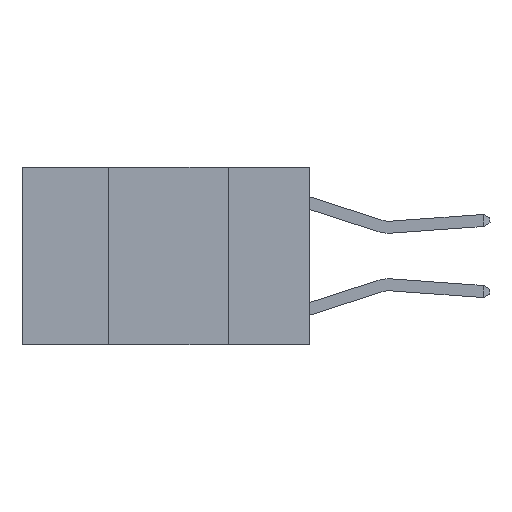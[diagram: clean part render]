
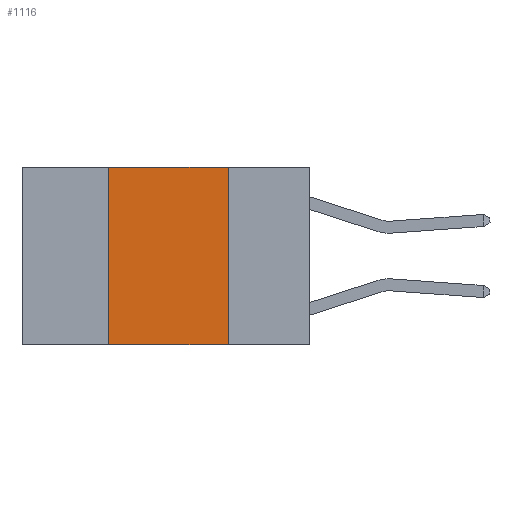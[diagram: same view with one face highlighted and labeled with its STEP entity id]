
A CAD part, left-side view. The second image highlights one B-rep face of the part: STEP entity #1116.
In plain terms, the highlighted planar face has unit normal (-1, 0, 0).
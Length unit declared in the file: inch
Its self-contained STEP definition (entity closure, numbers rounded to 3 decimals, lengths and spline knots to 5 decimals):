
#215 = CARTESIAN_POINT ( 'NONE',  ( 0., 0.6, 0. ) ) ;
#395 = FACE_OUTER_BOUND ( 'NONE', #25441, .T. ) ;
#673 = LINE ( 'NONE', #18969, #19925 ) ;
#1116 = ADVANCED_FACE ( 'NONE', ( #395 ), #12728, .F. ) ;
#1954 = CARTESIAN_POINT ( 'NONE',  ( 0., 0.42, 0. ) ) ;
#3042 = ORIENTED_EDGE ( 'NONE', *, *, #7827, .F. ) ;
#3159 = VECTOR ( 'NONE', #30495, 39.37008 ) ;
#4547 = DIRECTION ( 'NONE',  ( 0., 0., 1. ) ) ;
#6956 = VERTEX_POINT ( 'NONE', #14047 ) ;
#7087 = CARTESIAN_POINT ( 'NONE',  ( 0., 0.6, -0.37 ) ) ;
#7117 = CARTESIAN_POINT ( 'NONE',  ( 0., 0.17, 0. ) ) ;
#7827 = EDGE_CURVE ( 'NONE', #20014, #28870, #17836, .T. ) ;
#7899 = DIRECTION ( 'NONE',  ( 1., 0., 0. ) ) ;
#9595 = DIRECTION ( 'NONE',  ( 0., -1., 0. ) ) ;
#11465 = LINE ( 'NONE', #7087, #23945 ) ;
#12728 = PLANE ( 'NONE',  #18459 ) ;
#14047 = CARTESIAN_POINT ( 'NONE',  ( 0., 0.17, -0.37 ) ) ;
#15135 = CARTESIAN_POINT ( 'NONE',  ( 0., 0.42, -0.37 ) ) ;
#17836 = LINE ( 'NONE', #1954, #30318 ) ;
#18459 = AXIS2_PLACEMENT_3D ( 'NONE', #215, #7899, #25372 ) ;
#18969 = CARTESIAN_POINT ( 'NONE',  ( 0., 0.17, 0. ) ) ;
#19925 = VECTOR ( 'NONE', #29012, 39.37008 ) ;
#20014 = VERTEX_POINT ( 'NONE', #15135 ) ;
#22272 = ORIENTED_EDGE ( 'NONE', *, *, #31257, .F. ) ;
#23155 = LINE ( 'NONE', #27988, #3159 ) ;
#23511 = VERTEX_POINT ( 'NONE', #7117 ) ;
#23827 = ORIENTED_EDGE ( 'NONE', *, *, #26244, .T. ) ;
#23945 = VECTOR ( 'NONE', #9595, 39.37008 ) ;
#25372 = DIRECTION ( 'NONE',  ( 0., 0., -1. ) ) ;
#25441 = EDGE_LOOP ( 'NONE', ( #22272, #28912, #3042, #23827 ) ) ;
#26244 = EDGE_CURVE ( 'NONE', #20014, #6956, #11465, .T. ) ;
#27988 = CARTESIAN_POINT ( 'NONE',  ( 0., 0.6, 0. ) ) ;
#28870 = VERTEX_POINT ( 'NONE', #31525 ) ;
#28912 = ORIENTED_EDGE ( 'NONE', *, *, #29824, .F. ) ;
#29012 = DIRECTION ( 'NONE',  ( 0., 0., -1. ) ) ;
#29824 = EDGE_CURVE ( 'NONE', #28870, #23511, #23155, .T. ) ;
#30318 = VECTOR ( 'NONE', #4547, 39.37008 ) ;
#30495 = DIRECTION ( 'NONE',  ( 0., -1., 0. ) ) ;
#31257 = EDGE_CURVE ( 'NONE', #23511, #6956, #673, .T. ) ;
#31525 = CARTESIAN_POINT ( 'NONE',  ( 0., 0.42, 0. ) ) ;
